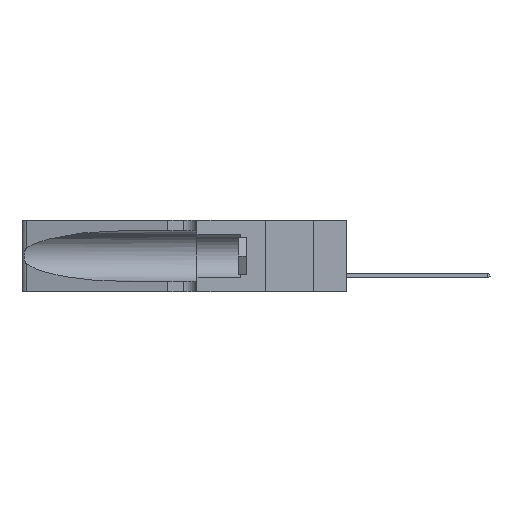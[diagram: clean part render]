
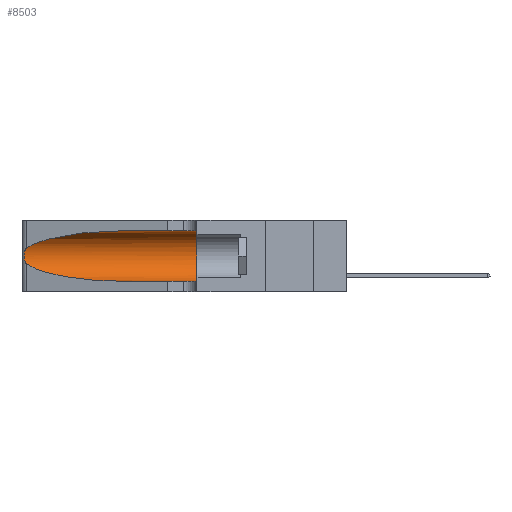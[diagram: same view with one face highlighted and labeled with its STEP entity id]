
A CAD part, left-side view. The second image highlights one B-rep face of the part: STEP entity #8503.
In plain terms, the highlighted cylindrical face has radius 3.308 mm (diameter 6.617 mm), a partial arc.
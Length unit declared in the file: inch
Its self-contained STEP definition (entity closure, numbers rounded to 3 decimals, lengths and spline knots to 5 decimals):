
#511 = CIRCLE ( 'NONE', #22997, 0.13025 ) ;
#774 = VERTEX_POINT ( 'NONE', #15479 ) ;
#792 = CARTESIAN_POINT ( 'NONE',  ( 0.25487, 1.22718, 0.14631 ) ) ;
#1041 = CARTESIAN_POINT ( 'NONE',  ( 0.25487, 1.22718, 0.22369 ) ) ;
#1429 = CARTESIAN_POINT ( 'NONE',  ( 0.25854, 1.2359, 0.20912 ) ) ;
#1550 = VERTEX_POINT ( 'NONE', #3901 ) ;
#1680 = VERTEX_POINT ( 'NONE', #792 ) ;
#1831 = ORIENTED_EDGE ( 'NONE', *, *, #12315, .T. ) ;
#2294 = CARTESIAN_POINT ( 'NONE',  ( 0.25487, 1.22718, 0.22369 ) ) ;
#2494 = EDGE_CURVE ( 'NONE', #5700, #22824, #10626, .T. ) ;
#2735 = VECTOR ( 'NONE', #15194, 39.37008 ) ;
#2778 =( BOUNDED_CURVE ( )  B_SPLINE_CURVE ( 3, ( #4618, #9916, #19056, #9845 ),
 .UNSPECIFIED., .F., .T. ) 
 B_SPLINE_CURVE_WITH_KNOTS ( ( 4, 4 ),
 ( 3.44316, 4.71239 ),
 .UNSPECIFIED. ) 
 CURVE ( )  GEOMETRIC_REPRESENTATION_ITEM ( )  RATIONAL_B_SPLINE_CURVE ( ( 1., 0.87, 0.87, 1. ) ) 
 REPRESENTATION_ITEM ( '' )  );
#3507 = FACE_OUTER_BOUND ( 'NONE', #22870, .T. ) ;
#3739 = CARTESIAN_POINT ( 'NONE',  ( 0.1305, 0.72297, 0.05475 ) ) ;
#3761 = CARTESIAN_POINT ( 'NONE',  ( 0.25789, 1.23486, 0.15765 ) ) ;
#3901 = CARTESIAN_POINT ( 'NONE',  ( 0.1305, 0.35, 0.05475 ) ) ;
#4294 = CARTESIAN_POINT ( 'NONE',  ( 0.1305, 1.61858, 0.185 ) ) ;
#4618 = CARTESIAN_POINT ( 'NONE',  ( 0.25487, 1.22718, 0.14631 ) ) ;
#5438 = EDGE_CURVE ( 'NONE', #774, #1550, #511, .T. ) ;
#5700 = VERTEX_POINT ( 'NONE', #22102 ) ;
#6071 = CARTESIAN_POINT ( 'NONE',  ( 0.1305, 1.61858, 0.31525 ) ) ;
#6528 = CARTESIAN_POINT ( 'NONE',  ( 0.1305, 0.35, 0.185 ) ) ;
#6760 = VECTOR ( 'NONE', #18691, 39.37008 ) ;
#8046 = B_SPLINE_CURVE_WITH_KNOTS ( 'NONE', 3,
 ( #17673, #17595, #10488, #23095, #1429, #10560, #23169, #12409, #21604, #9080, #3761, #21825, #13484, #17122 ),
 .UNSPECIFIED., .F., .F.,
 ( 4, 2, 2, 2, 2, 2, 4 ),
 ( 0., 0.00027, 0.00053, 0.00107, 0.0016, 0.00187, 0.00214 ),
 .UNSPECIFIED. ) ;
#8375 = DIRECTION ( 'NONE',  ( 0., 1., 0. ) ) ;
#8503 = ADVANCED_FACE ( 'NONE', ( #3507 ), #11141, .F. ) ;
#8712 = LINE ( 'NONE', #9126, #2735 ) ;
#9080 = CARTESIAN_POINT ( 'NONE',  ( 0.25856, 1.23593, 0.16098 ) ) ;
#9126 = CARTESIAN_POINT ( 'NONE',  ( 0.1305, 1.61858, 0.05475 ) ) ;
#9255 = ORIENTED_EDGE ( 'NONE', *, *, #23204, .T. ) ;
#9314 = ORIENTED_EDGE ( 'NONE', *, *, #2494, .T. ) ;
#9845 = CARTESIAN_POINT ( 'NONE',  ( 0.1305, 0.72297, 0.05475 ) ) ;
#9916 = CARTESIAN_POINT ( 'NONE',  ( 0.2373, 1.15595, 0.08982 ) ) ;
#10010 = CARTESIAN_POINT ( 'NONE',  ( 0.2373, 1.15595, 0.28018 ) ) ;
#10094 = DIRECTION ( 'NONE',  ( 0., 0., -1. ) ) ;
#10164 = CARTESIAN_POINT ( 'NONE',  ( 0.18966, 0.96281, 0.31525 ) ) ;
#10231 = ORIENTED_EDGE ( 'NONE', *, *, #5438, .F. ) ;
#10365 = AXIS2_PLACEMENT_3D ( 'NONE', #4294, #11228, #10094 ) ;
#10488 = CARTESIAN_POINT ( 'NONE',  ( 0.25639, 1.23184, 0.21858 ) ) ;
#10560 = CARTESIAN_POINT ( 'NONE',  ( 0.26018, 1.23835, 0.19895 ) ) ;
#10626 =( BOUNDED_CURVE ( )  B_SPLINE_CURVE ( 3, ( #15458, #10164, #10010, #1041 ),
 .UNSPECIFIED., .F., .F. ) 
 B_SPLINE_CURVE_WITH_KNOTS ( ( 4, 4 ),
 ( 1.5708, 2.84003 ),
 .UNSPECIFIED. ) 
 CURVE ( )  GEOMETRIC_REPRESENTATION_ITEM ( )  RATIONAL_B_SPLINE_CURVE ( ( 1., 0.87, 0.87, 1. ) ) 
 REPRESENTATION_ITEM ( '' )  );
#11141 = CYLINDRICAL_SURFACE ( 'NONE', #10365, 0.13025 ) ;
#11228 = DIRECTION ( 'NONE',  ( 0., -1., 0. ) ) ;
#12315 = EDGE_CURVE ( 'NONE', #19959, #1550, #8712, .T. ) ;
#12409 = CARTESIAN_POINT ( 'NONE',  ( 0.26075, 1.23896, 0.178 ) ) ;
#13484 = CARTESIAN_POINT ( 'NONE',  ( 0.25555, 1.22993, 0.14849 ) ) ;
#15194 = DIRECTION ( 'NONE',  ( 0., -1., 0. ) ) ;
#15259 = LINE ( 'NONE', #6071, #6760 ) ;
#15458 = CARTESIAN_POINT ( 'NONE',  ( 0.1305, 0.72297, 0.31525 ) ) ;
#15479 = CARTESIAN_POINT ( 'NONE',  ( 0.1305, 0.35, 0.31525 ) ) ;
#15621 = DIRECTION ( 'NONE',  ( 0., 0., 1. ) ) ;
#16168 = EDGE_CURVE ( 'NONE', #5700, #774, #15259, .T. ) ;
#17122 = CARTESIAN_POINT ( 'NONE',  ( 0.25487, 1.22718, 0.14631 ) ) ;
#17595 = CARTESIAN_POINT ( 'NONE',  ( 0.25555, 1.22994, 0.2215 ) ) ;
#17673 = CARTESIAN_POINT ( 'NONE',  ( 0.25487, 1.22718, 0.22369 ) ) ;
#18691 = DIRECTION ( 'NONE',  ( 0., -1., 0. ) ) ;
#19056 = CARTESIAN_POINT ( 'NONE',  ( 0.18966, 0.96281, 0.05475 ) ) ;
#19127 = EDGE_CURVE ( 'NONE', #22824, #1680, #8046, .T. ) ;
#19549 = ORIENTED_EDGE ( 'NONE', *, *, #19127, .T. ) ;
#19959 = VERTEX_POINT ( 'NONE', #3739 ) ;
#20817 = ORIENTED_EDGE ( 'NONE', *, *, #16168, .F. ) ;
#21604 = CARTESIAN_POINT ( 'NONE',  ( 0.26017, 1.23833, 0.17102 ) ) ;
#21825 = CARTESIAN_POINT ( 'NONE',  ( 0.25639, 1.23186, 0.15144 ) ) ;
#22102 = CARTESIAN_POINT ( 'NONE',  ( 0.1305, 0.72297, 0.31525 ) ) ;
#22824 = VERTEX_POINT ( 'NONE', #2294 ) ;
#22870 = EDGE_LOOP ( 'NONE', ( #9314, #19549, #9255, #1831, #10231, #20817 ) ) ;
#22997 = AXIS2_PLACEMENT_3D ( 'NONE', #6528, #8375, #15621 ) ;
#23095 = CARTESIAN_POINT ( 'NONE',  ( 0.25787, 1.23484, 0.2124 ) ) ;
#23169 = CARTESIAN_POINT ( 'NONE',  ( 0.26075, 1.23896, 0.19203 ) ) ;
#23204 = EDGE_CURVE ( 'NONE', #1680, #19959, #2778, .T. ) ;
